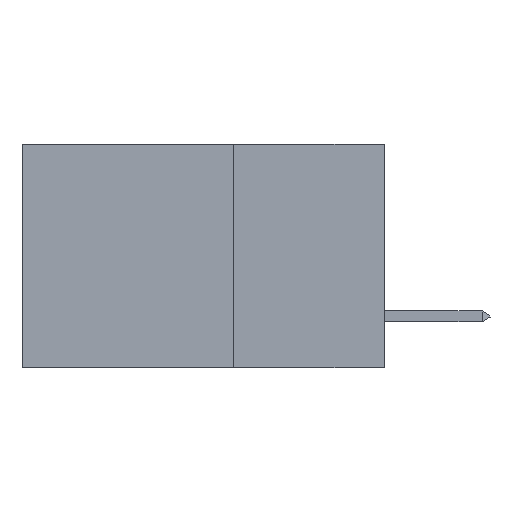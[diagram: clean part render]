
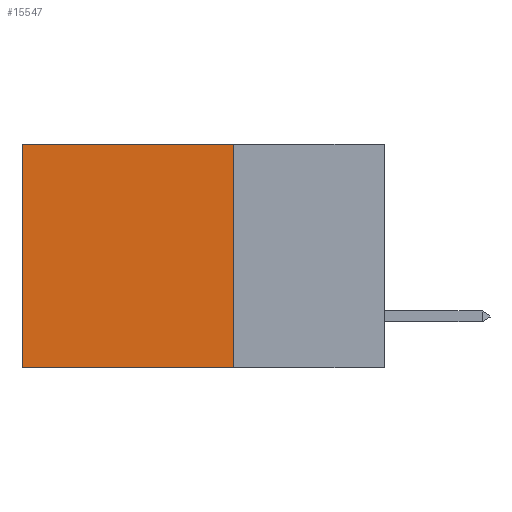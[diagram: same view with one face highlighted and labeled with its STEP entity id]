
A CAD part, left-side view. The second image highlights one B-rep face of the part: STEP entity #15547.
In plain terms, the highlighted planar face has unit normal (-1, 0, 0).
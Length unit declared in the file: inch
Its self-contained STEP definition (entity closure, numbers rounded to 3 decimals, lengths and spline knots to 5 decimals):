
#639 = EDGE_CURVE ( 'NONE', #21951, #7042, #10520, .T. ) ;
#1284 = VECTOR ( 'NONE', #3134, 39.37008 ) ;
#1723 = CARTESIAN_POINT ( 'NONE',  ( 0.2875, 0.25, 0. ) ) ;
#2427 = FACE_OUTER_BOUND ( 'NONE', #12994, .T. ) ;
#2745 = CARTESIAN_POINT ( 'NONE',  ( 0.2875, 0.25, -0.37 ) ) ;
#3128 = ORIENTED_EDGE ( 'NONE', *, *, #17880, .T. ) ;
#3134 = DIRECTION ( 'NONE',  ( 0., 1., 0. ) ) ;
#3173 = VECTOR ( 'NONE', #10615, 39.37008 ) ;
#3473 = DIRECTION ( 'NONE',  ( 0., 0., -1. ) ) ;
#3602 = ORIENTED_EDGE ( 'NONE', *, *, #16355, .F. ) ;
#4673 = DIRECTION ( 'NONE',  ( 0., 0., -1. ) ) ;
#5116 = LINE ( 'NONE', #1723, #5361 ) ;
#5361 = VECTOR ( 'NONE', #3473, 39.37008 ) ;
#6325 = LINE ( 'NONE', #19291, #16648 ) ;
#6680 = LINE ( 'NONE', #18545, #1284 ) ;
#7042 = VERTEX_POINT ( 'NONE', #16262 ) ;
#9336 = CARTESIAN_POINT ( 'NONE',  ( 0.2875, 0.6, -0.37 ) ) ;
#10520 = LINE ( 'NONE', #20925, #3173 ) ;
#10615 = DIRECTION ( 'NONE',  ( 0., 1., 0. ) ) ;
#11713 = VERTEX_POINT ( 'NONE', #2745 ) ;
#12994 = EDGE_LOOP ( 'NONE', ( #3128, #3602, #14862, #19135 ) ) ;
#13389 = PLANE ( 'NONE',  #17508 ) ;
#14862 = ORIENTED_EDGE ( 'NONE', *, *, #15745, .F. ) ;
#15314 = CARTESIAN_POINT ( 'NONE',  ( 0.2875, 0.25, 0. ) ) ;
#15547 = ADVANCED_FACE ( 'NONE', ( #2427 ), #13389, .F. ) ;
#15745 = EDGE_CURVE ( 'NONE', #21951, #11713, #5116, .T. ) ;
#16262 = CARTESIAN_POINT ( 'NONE',  ( 0.2875, 0.6, 0. ) ) ;
#16355 = EDGE_CURVE ( 'NONE', #11713, #18474, #6680, .T. ) ;
#16648 = VECTOR ( 'NONE', #19589, 39.37008 ) ;
#17508 = AXIS2_PLACEMENT_3D ( 'NONE', #22197, #22118, #4673 ) ;
#17880 = EDGE_CURVE ( 'NONE', #7042, #18474, #6325, .T. ) ;
#18474 = VERTEX_POINT ( 'NONE', #9336 ) ;
#18545 = CARTESIAN_POINT ( 'NONE',  ( 0.2875, 0.25, -0.37 ) ) ;
#19135 = ORIENTED_EDGE ( 'NONE', *, *, #639, .T. ) ;
#19291 = CARTESIAN_POINT ( 'NONE',  ( 0.2875, 0.6, 0. ) ) ;
#19589 = DIRECTION ( 'NONE',  ( 0., 0., -1. ) ) ;
#20925 = CARTESIAN_POINT ( 'NONE',  ( 0.2875, 0.25, 0. ) ) ;
#21951 = VERTEX_POINT ( 'NONE', #15314 ) ;
#22118 = DIRECTION ( 'NONE',  ( 1., 0., 0. ) ) ;
#22197 = CARTESIAN_POINT ( 'NONE',  ( 0.2875, 0.25, 0. ) ) ;
